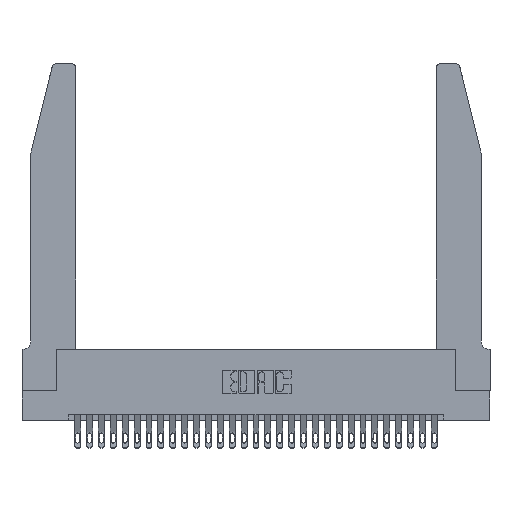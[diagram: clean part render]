
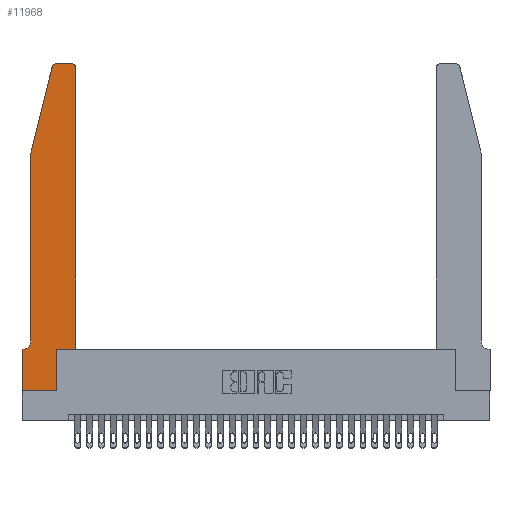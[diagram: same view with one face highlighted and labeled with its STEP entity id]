
A CAD part, top view. The second image highlights one B-rep face of the part: STEP entity #11968.
In plain terms, the highlighted planar face has unit normal (0, 0, 1).
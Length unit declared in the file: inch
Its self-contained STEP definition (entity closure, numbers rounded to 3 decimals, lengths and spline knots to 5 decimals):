
#108 = AXIS2_PLACEMENT_3D ( 'NONE', #6597, #15680, #15984 ) ;
#175 = LINE ( 'NONE', #14610, #21072 ) ;
#573 = ORIENTED_EDGE ( 'NONE', *, *, #11003, .T. ) ;
#726 = LINE ( 'NONE', #24821, #3706 ) ;
#1026 = CIRCLE ( 'NONE', #24945, 0.03 ) ;
#1412 = LINE ( 'NONE', #27360, #11488 ) ;
#1627 = VERTEX_POINT ( 'NONE', #3186 ) ;
#1717 = CARTESIAN_POINT ( 'NONE',  ( 0.2865, 0.35, 0.37 ) ) ;
#1989 = CARTESIAN_POINT ( 'NONE',  ( 0.4205, 2.72, 0.37 ) ) ;
#2120 = DIRECTION ( 'NONE',  ( -0.239, -0.971, 0. ) ) ;
#2148 = EDGE_CURVE ( 'NONE', #4431, #13251, #1026, .T. ) ;
#2432 = VERTEX_POINT ( 'NONE', #15301 ) ;
#2583 = VERTEX_POINT ( 'NONE', #11315 ) ;
#2817 = ORIENTED_EDGE ( 'NONE', *, *, #19734, .T. ) ;
#3186 = CARTESIAN_POINT ( 'NONE',  ( 0.4505, 2.72, 0.37 ) ) ;
#3301 = EDGE_CURVE ( 'NONE', #12243, #4431, #30420, .T. ) ;
#3706 = VECTOR ( 'NONE', #20229, 39.37008 ) ;
#3798 = EDGE_CURVE ( 'NONE', #6088, #11983, #175, .T. ) ;
#3849 = CARTESIAN_POINT ( 'NONE',  ( 0.0755, 2., 0.37 ) ) ;
#4167 = DIRECTION ( 'NONE',  ( 0., 0., 1. ) ) ;
#4431 = VERTEX_POINT ( 'NONE', #14528 ) ;
#4741 = CARTESIAN_POINT ( 'NONE',  ( 0.0755, 0.42, 0.37 ) ) ;
#5355 = VECTOR ( 'NONE', #10110, 39.37008 ) ;
#5576 = CARTESIAN_POINT ( 'NONE',  ( 0., 0., 0.37 ) ) ;
#5582 = VERTEX_POINT ( 'NONE', #12672 ) ;
#6088 = VERTEX_POINT ( 'NONE', #21313 ) ;
#6597 = CARTESIAN_POINT ( 'NONE',  ( 0., 0.35, 0.37 ) ) ;
#7554 = LINE ( 'NONE', #14099, #24362 ) ;
#7810 = ORIENTED_EDGE ( 'NONE', *, *, #3301, .T. ) ;
#8141 = ORIENTED_EDGE ( 'NONE', *, *, #19869, .T. ) ;
#8531 = VERTEX_POINT ( 'NONE', #3849 ) ;
#9290 = ORIENTED_EDGE ( 'NONE', *, *, #24740, .T. ) ;
#9414 = AXIS2_PLACEMENT_3D ( 'NONE', #1989, #4167, #25661 ) ;
#9465 = CARTESIAN_POINT ( 'NONE',  ( 0.0755, 2., 0.37 ) ) ;
#9738 = CIRCLE ( 'NONE', #9414, 0.03 ) ;
#10110 = DIRECTION ( 'NONE',  ( 1., 0., 0. ) ) ;
#10902 = CIRCLE ( 'NONE', #29418, 0.07 ) ;
#11003 = EDGE_CURVE ( 'NONE', #5582, #1627, #15076, .T. ) ;
#11315 = CARTESIAN_POINT ( 'NONE',  ( 0., 0.35, 0.37 ) ) ;
#11488 = VECTOR ( 'NONE', #25001, 39.37008 ) ;
#11753 = VECTOR ( 'NONE', #21724, 39.37008 ) ;
#11824 = CARTESIAN_POINT ( 'NONE',  ( 0., 0., 0.37 ) ) ;
#11968 = ADVANCED_FACE ( 'NONE', ( #15412 ), #23191, .T. ) ;
#11983 = VERTEX_POINT ( 'NONE', #1717 ) ;
#12216 = CARTESIAN_POINT ( 'NONE',  ( 0.4205, 2.75, 0.37 ) ) ;
#12243 = VERTEX_POINT ( 'NONE', #12216 ) ;
#12649 = ORIENTED_EDGE ( 'NONE', *, *, #2148, .T. ) ;
#12672 = CARTESIAN_POINT ( 'NONE',  ( 0.4505, 0.35, 0.37 ) ) ;
#12733 = DIRECTION ( 'NONE',  ( 0., 1., 0. ) ) ;
#12991 = CARTESIAN_POINT ( 'NONE',  ( 0.284, 2.72, 0.37 ) ) ;
#13251 = VERTEX_POINT ( 'NONE', #29432 ) ;
#14099 = CARTESIAN_POINT ( 'NONE',  ( 0.0755, 2., 0.37 ) ) ;
#14528 = CARTESIAN_POINT ( 'NONE',  ( 0.284, 2.75, 0.37 ) ) ;
#14565 = VECTOR ( 'NONE', #16451, 39.37008 ) ;
#14610 = CARTESIAN_POINT ( 'NONE',  ( 0.2865, 0.35, 0.37 ) ) ;
#15076 = LINE ( 'NONE', #16805, #27022 ) ;
#15282 = DIRECTION ( 'NONE',  ( 0., 0., -1. ) ) ;
#15301 = CARTESIAN_POINT ( 'NONE',  ( 0.0055, 0.35, 0.37 ) ) ;
#15412 = FACE_OUTER_BOUND ( 'NONE', #26524, .T. ) ;
#15680 = DIRECTION ( 'NONE',  ( 0., 0., 1. ) ) ;
#15984 = DIRECTION ( 'NONE',  ( 1., 0., 0. ) ) ;
#16056 = VERTEX_POINT ( 'NONE', #11824 ) ;
#16451 = DIRECTION ( 'NONE',  ( 0., -1., 0. ) ) ;
#16476 = DIRECTION ( 'NONE',  ( 0., 1., 0. ) ) ;
#16805 = CARTESIAN_POINT ( 'NONE',  ( 0.4505, 0.35, 0.37 ) ) ;
#17801 = DIRECTION ( 'NONE',  ( 1., 0., 0. ) ) ;
#17905 = DIRECTION ( 'NONE',  ( -1., 0., 0. ) ) ;
#18215 = ORIENTED_EDGE ( 'NONE', *, *, #29238, .T. ) ;
#18669 = ORIENTED_EDGE ( 'NONE', *, *, #25323, .T. ) ;
#18919 = CARTESIAN_POINT ( 'NONE',  ( 0.2605, 2.75, 0.37 ) ) ;
#19183 = EDGE_CURVE ( 'NONE', #16056, #6088, #23656, .T. ) ;
#19734 = EDGE_CURVE ( 'NONE', #2583, #16056, #22139, .T. ) ;
#19840 = ORIENTED_EDGE ( 'NONE', *, *, #19183, .T. ) ;
#19869 = EDGE_CURVE ( 'NONE', #21398, #2432, #10902, .T. ) ;
#20229 = DIRECTION ( 'NONE',  ( 1., 0., 0. ) ) ;
#21072 = VECTOR ( 'NONE', #12733, 39.37008 ) ;
#21313 = CARTESIAN_POINT ( 'NONE',  ( 0.2865, 0., 0.37 ) ) ;
#21398 = VERTEX_POINT ( 'NONE', #4741 ) ;
#21724 = DIRECTION ( 'NONE',  ( -1., 0., 0. ) ) ;
#22112 = CARTESIAN_POINT ( 'NONE',  ( 0., 0., 0.37 ) ) ;
#22139 = LINE ( 'NONE', #5576, #29219 ) ;
#23191 = PLANE ( 'NONE',  #108 ) ;
#23656 = LINE ( 'NONE', #22112, #5355 ) ;
#23858 = EDGE_CURVE ( 'NONE', #8531, #21398, #26874, .T. ) ;
#24362 = VECTOR ( 'NONE', #2120, 39.37008 ) ;
#24740 = EDGE_CURVE ( 'NONE', #11983, #5582, #726, .T. ) ;
#24821 = CARTESIAN_POINT ( 'NONE',  ( 0.4505, 0.35, 0.37 ) ) ;
#24945 = AXIS2_PLACEMENT_3D ( 'NONE', #12991, #29673, #17801 ) ;
#25001 = DIRECTION ( 'NONE',  ( -1., 0., 0. ) ) ;
#25007 = DIRECTION ( 'NONE',  ( 0., -1., 0. ) ) ;
#25323 = EDGE_CURVE ( 'NONE', #2432, #2583, #1412, .T. ) ;
#25661 = DIRECTION ( 'NONE',  ( 1., 0., 0. ) ) ;
#26304 = ORIENTED_EDGE ( 'NONE', *, *, #3798, .T. ) ;
#26524 = EDGE_LOOP ( 'NONE', ( #7810, #12649, #18215, #29722, #8141, #18669, #2817, #19840, #26304, #9290, #573, #29470 ) ) ;
#26874 = LINE ( 'NONE', #9465, #14565 ) ;
#27022 = VECTOR ( 'NONE', #16476, 39.37008 ) ;
#27166 = CARTESIAN_POINT ( 'NONE',  ( 0.0055, 0.42, 0.37 ) ) ;
#27360 = CARTESIAN_POINT ( 'NONE',  ( 0.0755, 0.35, 0.37 ) ) ;
#29219 = VECTOR ( 'NONE', #25007, 39.37008 ) ;
#29238 = EDGE_CURVE ( 'NONE', #13251, #8531, #7554, .T. ) ;
#29418 = AXIS2_PLACEMENT_3D ( 'NONE', #27166, #15282, #17905 ) ;
#29432 = CARTESIAN_POINT ( 'NONE',  ( 0.25487, 2.72718, 0.37 ) ) ;
#29470 = ORIENTED_EDGE ( 'NONE', *, *, #29858, .T. ) ;
#29673 = DIRECTION ( 'NONE',  ( 0., 0., 1. ) ) ;
#29722 = ORIENTED_EDGE ( 'NONE', *, *, #23858, .T. ) ;
#29858 = EDGE_CURVE ( 'NONE', #1627, #12243, #9738, .T. ) ;
#30420 = LINE ( 'NONE', #18919, #11753 ) ;
